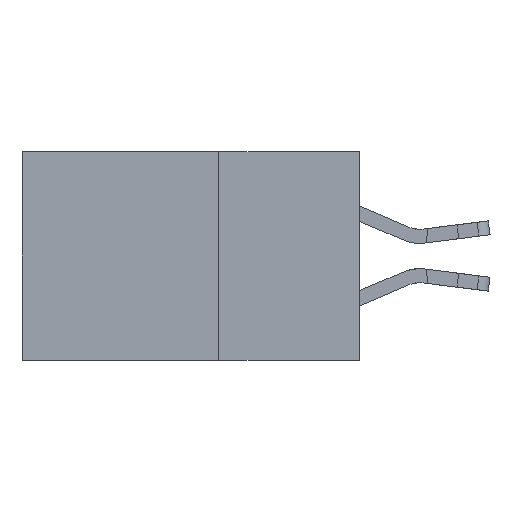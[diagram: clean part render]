
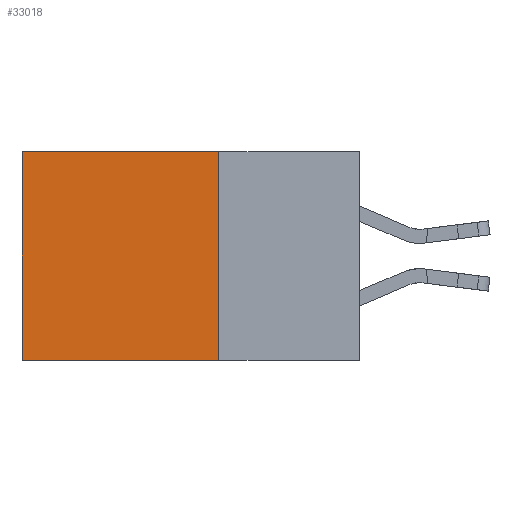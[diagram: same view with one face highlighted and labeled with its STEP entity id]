
A CAD part, left-side view. The second image highlights one B-rep face of the part: STEP entity #33018.
In plain terms, the highlighted planar face has unit normal (-1, 0, 0).
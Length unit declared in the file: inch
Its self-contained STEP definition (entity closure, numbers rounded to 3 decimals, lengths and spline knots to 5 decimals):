
#544 = VERTEX_POINT ( 'NONE', #33110 ) ;
#3408 = FACE_OUTER_BOUND ( 'NONE', #28192, .T. ) ;
#4311 = CARTESIAN_POINT ( 'NONE',  ( 0.2875, 0.25, -0.37 ) ) ;
#5849 = VECTOR ( 'NONE', #14861, 39.37008 ) ;
#6718 = VECTOR ( 'NONE', #25538, 39.37008 ) ;
#6762 = CARTESIAN_POINT ( 'NONE',  ( 0.2875, 0.25, 0. ) ) ;
#7189 = ORIENTED_EDGE ( 'NONE', *, *, #18444, .F. ) ;
#7706 = EDGE_CURVE ( 'NONE', #19005, #9822, #30227, .T. ) ;
#8005 = CARTESIAN_POINT ( 'NONE',  ( 0.2875, 0.6, -0.37 ) ) ;
#9143 = DIRECTION ( 'NONE',  ( 1., 0., 0. ) ) ;
#9324 = ORIENTED_EDGE ( 'NONE', *, *, #23474, .T. ) ;
#9822 = VERTEX_POINT ( 'NONE', #17974 ) ;
#9864 = CARTESIAN_POINT ( 'NONE',  ( 0.2875, 0.25, 0. ) ) ;
#11599 = DIRECTION ( 'NONE',  ( 0., 1., 0. ) ) ;
#11941 = CARTESIAN_POINT ( 'NONE',  ( 0.2875, 0.25, 0. ) ) ;
#13664 = LINE ( 'NONE', #24287, #5849 ) ;
#14365 = ORIENTED_EDGE ( 'NONE', *, *, #31309, .F. ) ;
#14861 = DIRECTION ( 'NONE',  ( 0., 0., -1. ) ) ;
#17140 = CARTESIAN_POINT ( 'NONE',  ( 0.2875, 0.25, 0. ) ) ;
#17899 = AXIS2_PLACEMENT_3D ( 'NONE', #17140, #9143, #22184 ) ;
#17974 = CARTESIAN_POINT ( 'NONE',  ( 0.2875, 0.6, 0. ) ) ;
#18444 = EDGE_CURVE ( 'NONE', #19005, #544, #30622, .T. ) ;
#19005 = VERTEX_POINT ( 'NONE', #9864 ) ;
#19997 = DIRECTION ( 'NONE',  ( 0., 0., -1. ) ) ;
#22184 = DIRECTION ( 'NONE',  ( 0., 0., -1. ) ) ;
#23474 = EDGE_CURVE ( 'NONE', #9822, #24268, #13664, .T. ) ;
#23628 = VECTOR ( 'NONE', #19997, 39.37008 ) ;
#23903 = ORIENTED_EDGE ( 'NONE', *, *, #7706, .T. ) ;
#24268 = VERTEX_POINT ( 'NONE', #8005 ) ;
#24287 = CARTESIAN_POINT ( 'NONE',  ( 0.2875, 0.6, 0. ) ) ;
#24809 = PLANE ( 'NONE',  #17899 ) ;
#25538 = DIRECTION ( 'NONE',  ( 0., 1., 0. ) ) ;
#28149 = LINE ( 'NONE', #4311, #6718 ) ;
#28192 = EDGE_LOOP ( 'NONE', ( #9324, #14365, #7189, #23903 ) ) ;
#30227 = LINE ( 'NONE', #11941, #30981 ) ;
#30622 = LINE ( 'NONE', #6762, #23628 ) ;
#30981 = VECTOR ( 'NONE', #11599, 39.37008 ) ;
#31309 = EDGE_CURVE ( 'NONE', #544, #24268, #28149, .T. ) ;
#33018 = ADVANCED_FACE ( 'NONE', ( #3408 ), #24809, .F. ) ;
#33110 = CARTESIAN_POINT ( 'NONE',  ( 0.2875, 0.25, -0.37 ) ) ;
